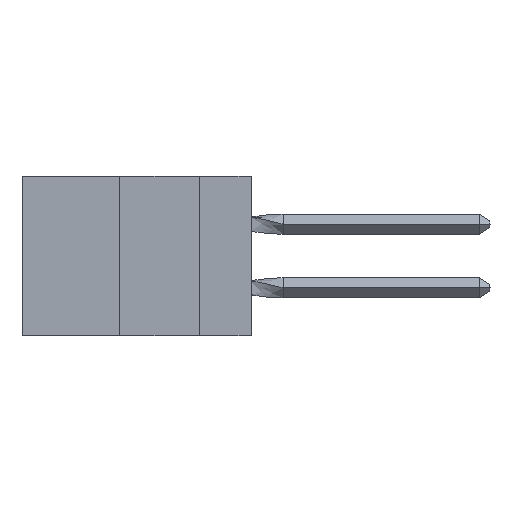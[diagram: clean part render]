
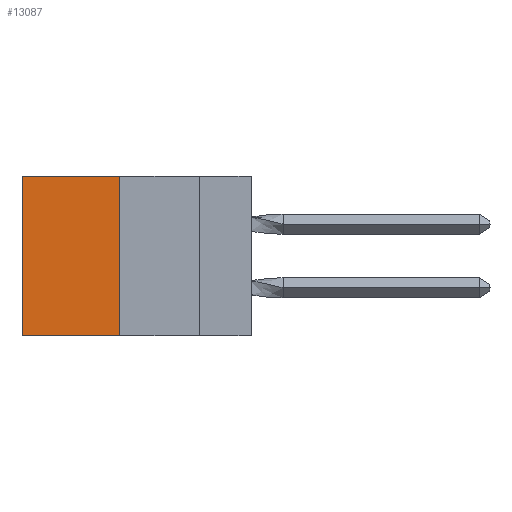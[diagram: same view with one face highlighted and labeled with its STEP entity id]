
A CAD part, left-side view. The second image highlights one B-rep face of the part: STEP entity #13087.
In plain terms, the highlighted planar face has unit normal (-1, 0, 0).
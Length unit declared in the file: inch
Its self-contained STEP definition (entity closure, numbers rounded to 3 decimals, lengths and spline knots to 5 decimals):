
#910 = DIRECTION ( 'NONE',  ( 0., 0., -1. ) ) ;
#1158 = EDGE_CURVE ( 'NONE', #8642, #3510, #13476, .T. ) ;
#2544 = CARTESIAN_POINT ( 'NONE',  ( 0.305, 0.72, -0.5 ) ) ;
#2761 = EDGE_CURVE ( 'NONE', #7167, #10571, #13248, .T. ) ;
#2849 = FACE_OUTER_BOUND ( 'NONE', #8759, .T. ) ;
#3452 = VECTOR ( 'NONE', #910, 39.37008 ) ;
#3510 = VERTEX_POINT ( 'NONE', #5742 ) ;
#4378 = CARTESIAN_POINT ( 'NONE',  ( 0.305, 0.413, -0.5 ) ) ;
#4426 = DIRECTION ( 'NONE',  ( 0., 1., 0. ) ) ;
#4704 = DIRECTION ( 'NONE',  ( 0., 0., -1. ) ) ;
#5294 = CARTESIAN_POINT ( 'NONE',  ( 0.305, 0.413, -0.5 ) ) ;
#5433 = CARTESIAN_POINT ( 'NONE',  ( 0.305, 0.72, 0. ) ) ;
#5559 = PLANE ( 'NONE',  #10941 ) ;
#5742 = CARTESIAN_POINT ( 'NONE',  ( 0.305, 0.72, -0.5 ) ) ;
#6634 = ORIENTED_EDGE ( 'NONE', *, *, #8054, .F. ) ;
#7167 = VERTEX_POINT ( 'NONE', #9392 ) ;
#7418 = VECTOR ( 'NONE', #8692, 39.37008 ) ;
#7600 = CARTESIAN_POINT ( 'NONE',  ( 0.305, 0.413, 0. ) ) ;
#7993 = DIRECTION ( 'NONE',  ( 1., 0., 0. ) ) ;
#8054 = EDGE_CURVE ( 'NONE', #10571, #3510, #10000, .T. ) ;
#8642 = VERTEX_POINT ( 'NONE', #5433 ) ;
#8692 = DIRECTION ( 'NONE',  ( 0., 1., 0. ) ) ;
#8759 = EDGE_LOOP ( 'NONE', ( #11896, #6634, #10208, #11061 ) ) ;
#9392 = CARTESIAN_POINT ( 'NONE',  ( 0.305, 0.413, 0. ) ) ;
#10000 = LINE ( 'NONE', #4378, #13526 ) ;
#10078 = CARTESIAN_POINT ( 'NONE',  ( 0.305, 0.413, -0.5 ) ) ;
#10208 = ORIENTED_EDGE ( 'NONE', *, *, #2761, .F. ) ;
#10571 = VERTEX_POINT ( 'NONE', #11280 ) ;
#10623 = VECTOR ( 'NONE', #12326, 39.37008 ) ;
#10941 = AXIS2_PLACEMENT_3D ( 'NONE', #10078, #7993, #4704 ) ;
#11061 = ORIENTED_EDGE ( 'NONE', *, *, #13836, .T. ) ;
#11280 = CARTESIAN_POINT ( 'NONE',  ( 0.305, 0.413, -0.5 ) ) ;
#11896 = ORIENTED_EDGE ( 'NONE', *, *, #1158, .T. ) ;
#12326 = DIRECTION ( 'NONE',  ( 0., 0., -1. ) ) ;
#13087 = ADVANCED_FACE ( 'NONE', ( #2849 ), #5559, .F. ) ;
#13165 = LINE ( 'NONE', #7600, #7418 ) ;
#13248 = LINE ( 'NONE', #5294, #3452 ) ;
#13476 = LINE ( 'NONE', #2544, #10623 ) ;
#13526 = VECTOR ( 'NONE', #4426, 39.37008 ) ;
#13836 = EDGE_CURVE ( 'NONE', #7167, #8642, #13165, .T. ) ;
